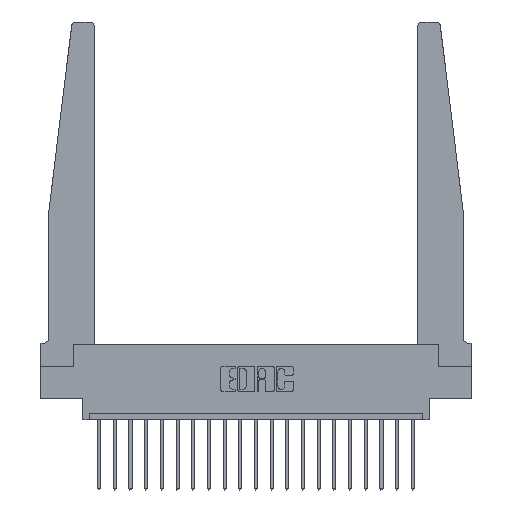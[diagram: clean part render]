
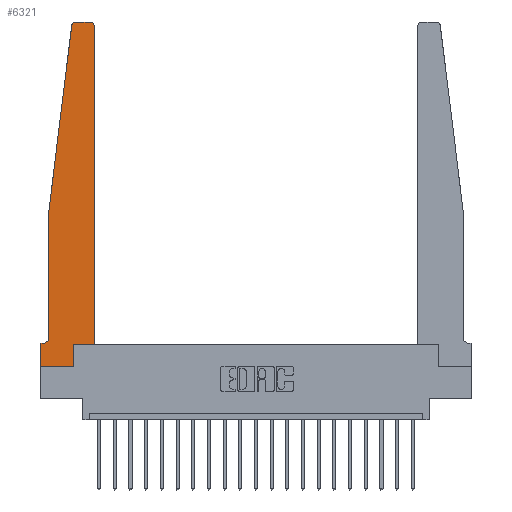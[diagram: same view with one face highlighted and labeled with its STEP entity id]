
A CAD part, top view. The second image highlights one B-rep face of the part: STEP entity #6321.
In plain terms, the highlighted planar face has unit normal (0, 0, 1).
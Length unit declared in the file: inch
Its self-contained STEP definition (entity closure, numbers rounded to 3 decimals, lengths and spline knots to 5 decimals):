
#274 = ORIENTED_EDGE ( 'NONE', *, *, #8058, .T. ) ;
#362 = CARTESIAN_POINT ( 'NONE',  ( 0., 0., 0.37 ) ) ;
#544 = CARTESIAN_POINT ( 'NONE',  ( 0.065, 0.1875, 0.37 ) ) ;
#732 = CARTESIAN_POINT ( 'NONE',  ( 0.015, 0.2375, 0.37 ) ) ;
#738 = VERTEX_POINT ( 'NONE', #14114 ) ;
#979 = ORIENTED_EDGE ( 'NONE', *, *, #6837, .T. ) ;
#1129 = EDGE_CURVE ( 'NONE', #738, #11121, #14858, .T. ) ;
#1659 = DIRECTION ( 'NONE',  ( 0., 1., 0. ) ) ;
#1669 = LINE ( 'NONE', #13265, #5230 ) ;
#2242 = VECTOR ( 'NONE', #11570, 39.37008 ) ;
#2511 = VERTEX_POINT ( 'NONE', #8315 ) ;
#2781 = DIRECTION ( 'NONE',  ( -0.122, -0.992, 0. ) ) ;
#2829 = ORIENTED_EDGE ( 'NONE', *, *, #10839, .T. ) ;
#2874 = VECTOR ( 'NONE', #16067, 39.37008 ) ;
#3061 = VERTEX_POINT ( 'NONE', #17467 ) ;
#3168 = EDGE_CURVE ( 'NONE', #11995, #6498, #9640, .T. ) ;
#3208 = LINE ( 'NONE', #9742, #12536 ) ;
#3288 = EDGE_CURVE ( 'NONE', #6498, #17150, #3208, .T. ) ;
#3555 = AXIS2_PLACEMENT_3D ( 'NONE', #18830, #16894, #15373 ) ;
#3726 = AXIS2_PLACEMENT_3D ( 'NONE', #732, #18975, #10921 ) ;
#4161 = DIRECTION ( 'NONE',  ( 0., 0., 1. ) ) ;
#4274 = CARTESIAN_POINT ( 'NONE',  ( 0.2605, 0.18, 0.37 ) ) ;
#4677 = EDGE_CURVE ( 'NONE', #18764, #2511, #1669, .T. ) ;
#5230 = VECTOR ( 'NONE', #6817, 39.37008 ) ;
#5237 = PLANE ( 'NONE',  #14243 ) ;
#5302 = LINE ( 'NONE', #362, #15538 ) ;
#5340 = FACE_OUTER_BOUND ( 'NONE', #19248, .T. ) ;
#5376 = DIRECTION ( 'NONE',  ( -1., 0., 0. ) ) ;
#5933 = VERTEX_POINT ( 'NONE', #13119 ) ;
#6291 = VECTOR ( 'NONE', #10018, 39.37008 ) ;
#6321 = ADVANCED_FACE ( 'NONE', ( #5340 ), #5237, .T. ) ;
#6478 = CARTESIAN_POINT ( 'NONE',  ( 0.425, 2.72, 0.37 ) ) ;
#6498 = VERTEX_POINT ( 'NONE', #7467 ) ;
#6586 = CARTESIAN_POINT ( 'NONE',  ( 0.25, 2.75, 0.37 ) ) ;
#6641 = VERTEX_POINT ( 'NONE', #12721 ) ;
#6683 = ORIENTED_EDGE ( 'NONE', *, *, #10893, .T. ) ;
#6817 = DIRECTION ( 'NONE',  ( 1., 0., 0. ) ) ;
#6837 = EDGE_CURVE ( 'NONE', #2511, #11995, #21200, .T. ) ;
#6861 = VECTOR ( 'NONE', #1659, 39.37008 ) ;
#7467 = CARTESIAN_POINT ( 'NONE',  ( 0.425, 0.18, 0.37 ) ) ;
#7644 = CARTESIAN_POINT ( 'NONE',  ( 0.065, 0.2375, 0.37 ) ) ;
#7707 = LINE ( 'NONE', #17466, #11472 ) ;
#8046 = DIRECTION ( 'NONE',  ( 0., 0., 1. ) ) ;
#8058 = EDGE_CURVE ( 'NONE', #11121, #6641, #7707, .T. ) ;
#8097 = EDGE_CURVE ( 'NONE', #6641, #11273, #18113, .T. ) ;
#8176 = AXIS2_PLACEMENT_3D ( 'NONE', #15527, #4161, #17254 ) ;
#8315 = CARTESIAN_POINT ( 'NONE',  ( 0.2605, 0., 0.37 ) ) ;
#8450 = CARTESIAN_POINT ( 'NONE',  ( 0.425, 0.18, 0.37 ) ) ;
#8743 = ORIENTED_EDGE ( 'NONE', *, *, #15144, .T. ) ;
#8826 = CARTESIAN_POINT ( 'NONE',  ( 0.24675, 2.72367, 0.37 ) ) ;
#9640 = LINE ( 'NONE', #8450, #2242 ) ;
#9742 = CARTESIAN_POINT ( 'NONE',  ( 0.425, 0.18, 0.37 ) ) ;
#9848 = CARTESIAN_POINT ( 'NONE',  ( 0.065, 1.25, 0.37 ) ) ;
#9862 = ORIENTED_EDGE ( 'NONE', *, *, #3168, .T. ) ;
#10018 = DIRECTION ( 'NONE',  ( -1., 0., 0. ) ) ;
#10839 = EDGE_CURVE ( 'NONE', #11273, #5933, #19839, .T. ) ;
#10893 = EDGE_CURVE ( 'NONE', #17150, #3061, #12291, .T. ) ;
#10921 = DIRECTION ( 'NONE',  ( -1., 0., 0. ) ) ;
#11121 = VERTEX_POINT ( 'NONE', #8826 ) ;
#11273 = VERTEX_POINT ( 'NONE', #7644 ) ;
#11472 = VECTOR ( 'NONE', #2781, 39.37008 ) ;
#11570 = DIRECTION ( 'NONE',  ( 1., 0., 0. ) ) ;
#11839 = ORIENTED_EDGE ( 'NONE', *, *, #18844, .T. ) ;
#11852 = CARTESIAN_POINT ( 'NONE',  ( 0., 0., 0.37 ) ) ;
#11995 = VERTEX_POINT ( 'NONE', #4274 ) ;
#12291 = CIRCLE ( 'NONE', #8176, 0.03 ) ;
#12536 = VECTOR ( 'NONE', #12964, 39.37008 ) ;
#12721 = CARTESIAN_POINT ( 'NONE',  ( 0.065, 1.25, 0.37 ) ) ;
#12775 = ORIENTED_EDGE ( 'NONE', *, *, #18629, .T. ) ;
#12964 = DIRECTION ( 'NONE',  ( 0., 1., 0. ) ) ;
#13119 = CARTESIAN_POINT ( 'NONE',  ( 0.015, 0.1875, 0.37 ) ) ;
#13265 = CARTESIAN_POINT ( 'NONE',  ( 0., 0., 0.37 ) ) ;
#13485 = CARTESIAN_POINT ( 'NONE',  ( 0., 0.1875, 0.37 ) ) ;
#13625 = ORIENTED_EDGE ( 'NONE', *, *, #1129, .T. ) ;
#13632 = CARTESIAN_POINT ( 'NONE',  ( 0., 0.1875, 0.37 ) ) ;
#13656 = DIRECTION ( 'NONE',  ( 0., -1., 0. ) ) ;
#14114 = CARTESIAN_POINT ( 'NONE',  ( 0.27653, 2.75, 0.37 ) ) ;
#14243 = AXIS2_PLACEMENT_3D ( 'NONE', #13485, #8046, #20050 ) ;
#14858 = CIRCLE ( 'NONE', #3555, 0.03 ) ;
#14913 = LINE ( 'NONE', #544, #17161 ) ;
#15128 = ORIENTED_EDGE ( 'NONE', *, *, #4677, .T. ) ;
#15144 = EDGE_CURVE ( 'NONE', #5933, #19181, #14913, .T. ) ;
#15373 = DIRECTION ( 'NONE',  ( 1., 0., 0. ) ) ;
#15498 = ORIENTED_EDGE ( 'NONE', *, *, #8097, .T. ) ;
#15527 = CARTESIAN_POINT ( 'NONE',  ( 0.395, 2.72, 0.37 ) ) ;
#15538 = VECTOR ( 'NONE', #13656, 39.37008 ) ;
#15705 = ORIENTED_EDGE ( 'NONE', *, *, #3288, .T. ) ;
#16067 = DIRECTION ( 'NONE',  ( 0., -1., 0. ) ) ;
#16366 = CARTESIAN_POINT ( 'NONE',  ( 0.2605, 0.18, 0.37 ) ) ;
#16676 = LINE ( 'NONE', #6586, #6291 ) ;
#16894 = DIRECTION ( 'NONE',  ( 0., 0., 1. ) ) ;
#17150 = VERTEX_POINT ( 'NONE', #6478 ) ;
#17161 = VECTOR ( 'NONE', #5376, 39.37008 ) ;
#17254 = DIRECTION ( 'NONE',  ( 1., 0., 0. ) ) ;
#17466 = CARTESIAN_POINT ( 'NONE',  ( 0.065, 1.25, 0.37 ) ) ;
#17467 = CARTESIAN_POINT ( 'NONE',  ( 0.395, 2.75, 0.37 ) ) ;
#18113 = LINE ( 'NONE', #9848, #2874 ) ;
#18629 = EDGE_CURVE ( 'NONE', #3061, #738, #16676, .T. ) ;
#18764 = VERTEX_POINT ( 'NONE', #11852 ) ;
#18830 = CARTESIAN_POINT ( 'NONE',  ( 0.27653, 2.72, 0.37 ) ) ;
#18844 = EDGE_CURVE ( 'NONE', #19181, #18764, #5302, .T. ) ;
#18975 = DIRECTION ( 'NONE',  ( 0., 0., -1. ) ) ;
#19181 = VERTEX_POINT ( 'NONE', #13632 ) ;
#19248 = EDGE_LOOP ( 'NONE', ( #12775, #13625, #274, #15498, #2829, #8743, #11839, #15128, #979, #9862, #15705, #6683 ) ) ;
#19839 = CIRCLE ( 'NONE', #3726, 0.05 ) ;
#20050 = DIRECTION ( 'NONE',  ( 1., 0., 0. ) ) ;
#21200 = LINE ( 'NONE', #16366, #6861 ) ;
